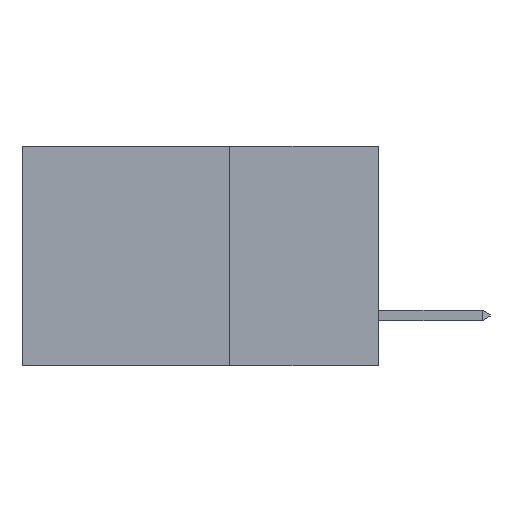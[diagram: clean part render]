
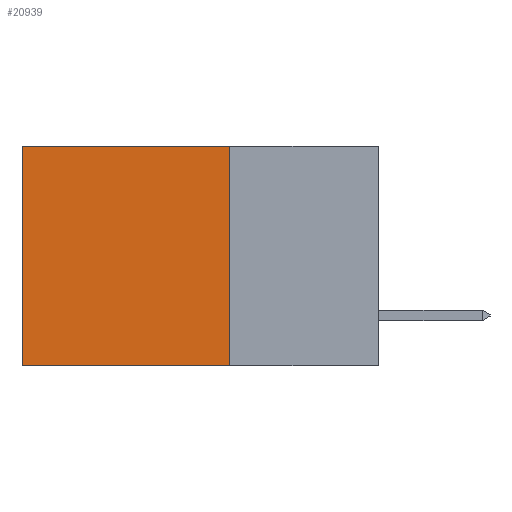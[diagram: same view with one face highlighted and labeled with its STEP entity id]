
A CAD part, left-side view. The second image highlights one B-rep face of the part: STEP entity #20939.
In plain terms, the highlighted planar face has unit normal (-1, 0, 0).
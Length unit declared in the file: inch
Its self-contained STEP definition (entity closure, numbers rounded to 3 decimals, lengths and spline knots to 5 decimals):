
#337 = ORIENTED_EDGE ( 'NONE', *, *, #24241, .T. ) ;
#3149 = CARTESIAN_POINT ( 'NONE',  ( 0.2615, 0.25, 0. ) ) ;
#4312 = PLANE ( 'NONE',  #6973 ) ;
#4352 = VERTEX_POINT ( 'NONE', #6982 ) ;
#4833 = ORIENTED_EDGE ( 'NONE', *, *, #20615, .F. ) ;
#5521 = CARTESIAN_POINT ( 'NONE',  ( 0.2615, 0.25, -0.37 ) ) ;
#5867 = LINE ( 'NONE', #23082, #15735 ) ;
#6273 = CARTESIAN_POINT ( 'NONE',  ( 0.2615, 0.6, -0.37 ) ) ;
#6703 = EDGE_CURVE ( 'NONE', #8335, #4352, #16207, .T. ) ;
#6970 = VERTEX_POINT ( 'NONE', #3149 ) ;
#6973 = AXIS2_PLACEMENT_3D ( 'NONE', #20004, #20086, #8298 ) ;
#6982 = CARTESIAN_POINT ( 'NONE',  ( 0.2615, 0.6, -0.37 ) ) ;
#7525 = DIRECTION ( 'NONE',  ( 0., 1., 0. ) ) ;
#7945 = VECTOR ( 'NONE', #7525, 39.37008 ) ;
#8298 = DIRECTION ( 'NONE',  ( 0., 0., -1. ) ) ;
#8335 = VERTEX_POINT ( 'NONE', #15033 ) ;
#8563 = LINE ( 'NONE', #23163, #18998 ) ;
#8790 = VERTEX_POINT ( 'NONE', #18275 ) ;
#9992 = ORIENTED_EDGE ( 'NONE', *, *, #6703, .T. ) ;
#10691 = EDGE_LOOP ( 'NONE', ( #9992, #12012, #4833, #337 ) ) ;
#12012 = ORIENTED_EDGE ( 'NONE', *, *, #24249, .F. ) ;
#15033 = CARTESIAN_POINT ( 'NONE',  ( 0.2615, 0.6, 0. ) ) ;
#15606 = VECTOR ( 'NONE', #20064, 39.37008 ) ;
#15735 = VECTOR ( 'NONE', #21033, 39.37008 ) ;
#16207 = LINE ( 'NONE', #6273, #15606 ) ;
#18275 = CARTESIAN_POINT ( 'NONE',  ( 0.2615, 0.25, -0.37 ) ) ;
#18998 = VECTOR ( 'NONE', #25126, 39.37008 ) ;
#20004 = CARTESIAN_POINT ( 'NONE',  ( 0.2615, 0.25, -0.37 ) ) ;
#20064 = DIRECTION ( 'NONE',  ( 0., 0., -1. ) ) ;
#20086 = DIRECTION ( 'NONE',  ( 1., 0., 0. ) ) ;
#20615 = EDGE_CURVE ( 'NONE', #6970, #8790, #5867, .T. ) ;
#20939 = ADVANCED_FACE ( 'NONE', ( #23379 ), #4312, .F. ) ;
#21033 = DIRECTION ( 'NONE',  ( 0., 0., -1. ) ) ;
#23082 = CARTESIAN_POINT ( 'NONE',  ( 0.2615, 0.25, -0.37 ) ) ;
#23163 = CARTESIAN_POINT ( 'NONE',  ( 0.2615, 0.25, 0. ) ) ;
#23379 = FACE_OUTER_BOUND ( 'NONE', #10691, .T. ) ;
#23603 = LINE ( 'NONE', #5521, #7945 ) ;
#24241 = EDGE_CURVE ( 'NONE', #6970, #8335, #8563, .T. ) ;
#24249 = EDGE_CURVE ( 'NONE', #8790, #4352, #23603, .T. ) ;
#25126 = DIRECTION ( 'NONE',  ( 0., 1., 0. ) ) ;
